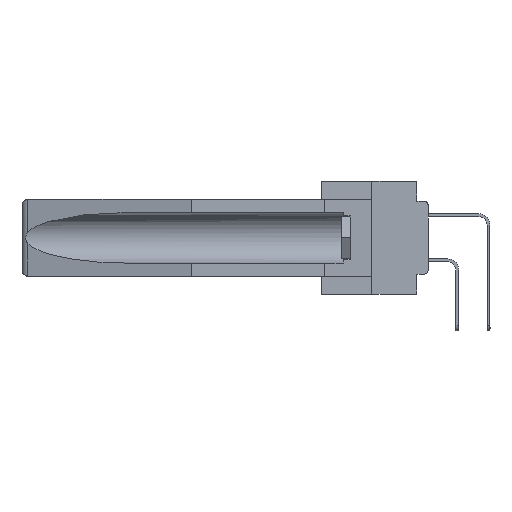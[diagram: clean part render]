
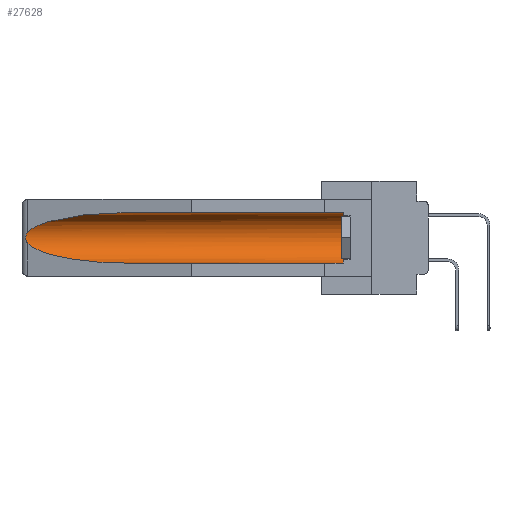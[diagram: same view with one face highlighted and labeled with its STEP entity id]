
A CAD part, left-side view. The second image highlights one B-rep face of the part: STEP entity #27628.
In plain terms, the highlighted cylindrical face has radius 2.857 mm (diameter 5.715 mm), a partial arc.
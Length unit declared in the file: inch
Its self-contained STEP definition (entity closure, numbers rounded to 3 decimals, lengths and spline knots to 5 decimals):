
#10 = ORIENTED_EDGE ( 'NONE', *, *, #17261, .T. ) ;
#563 = CARTESIAN_POINT ( 'NONE',  ( 0.155, -0.30754, -0.059 ) ) ;
#774 = EDGE_CURVE ( 'NONE', #17268, #7400, #1873, .T. ) ;
#1024 = DIRECTION ( 'NONE',  ( 0., 0., 1. ) ) ;
#1674 = CARTESIAN_POINT ( 'NONE',  ( 0.2673, 1.5327, -0.16383 ) ) ;
#1708 = AXIS2_PLACEMENT_3D ( 'NONE', #20218, #1818, #14169 ) ;
#1818 = DIRECTION ( 'NONE',  ( 0., 1., 0. ) ) ;
#1873 =( BOUNDED_CURVE ( )  B_SPLINE_CURVE ( 3, ( #21842, #6467, #18656, #9145 ),
 .UNSPECIFIED., .F., .F. ) 
 B_SPLINE_CURVE_WITH_KNOTS ( ( 4, 4 ),
 ( 4.71239, 6.08839 ),
 .UNSPECIFIED. ) 
 CURVE ( )  GEOMETRIC_REPRESENTATION_ITEM ( )  RATIONAL_B_SPLINE_CURVE ( ( 1., 0.848, 0.848, 1. ) ) 
 REPRESENTATION_ITEM ( '' )  );
#3133 = B_SPLINE_CURVE_WITH_KNOTS ( 'NONE', 3,
 ( #7586, #35607, #32234, #1674, #17251, #38547, #13736, #23155, #4782, #26237 ),
 .UNSPECIFIED., .F., .F.,
 ( 4, 2, 2, 2, 4 ),
 ( 0., 0.00029, 0.00058, 0.00087, 0.00117 ),
 .UNSPECIFIED. ) ;
#3295 = DIRECTION ( 'NONE',  ( 0., 1., 0. ) ) ;
#4119 = CARTESIAN_POINT ( 'NONE',  ( 0.155, 1.07973, -0.059 ) ) ;
#4595 = CARTESIAN_POINT ( 'NONE',  ( 0.155, 1.07973, -0.284 ) ) ;
#4782 = CARTESIAN_POINT ( 'NONE',  ( 0.26597, 1.5296, -0.19026 ) ) ;
#6467 = CARTESIAN_POINT ( 'NONE',  ( 0.21114, 1.30732, -0.059 ) ) ;
#6481 = EDGE_CURVE ( 'NONE', #9315, #17268, #15022, .T. ) ;
#6976 = EDGE_CURVE ( 'NONE', #22000, #14527, #27498, .T. ) ;
#7400 = VERTEX_POINT ( 'NONE', #12946 ) ;
#7586 = CARTESIAN_POINT ( 'NONE',  ( 0.26537, 1.52718, -0.14972 ) ) ;
#8863 = CARTESIAN_POINT ( 'NONE',  ( 0.26537, 1.52718, -0.19328 ) ) ;
#9120 = CARTESIAN_POINT ( 'NONE',  ( 0.155, 1.07973, -0.284 ) ) ;
#9145 = CARTESIAN_POINT ( 'NONE',  ( 0.26537, 1.52718, -0.14972 ) ) ;
#9315 = VERTEX_POINT ( 'NONE', #24206 ) ;
#12233 = ORIENTED_EDGE ( 'NONE', *, *, #31463, .T. ) ;
#12946 = CARTESIAN_POINT ( 'NONE',  ( 0.26537, 1.52718, -0.14972 ) ) ;
#13736 = CARTESIAN_POINT ( 'NONE',  ( 0.2673, 1.53269, -0.17917 ) ) ;
#14034 = VECTOR ( 'NONE', #3295, 39.37008 ) ;
#14169 = DIRECTION ( 'NONE',  ( 0., 0., 1. ) ) ;
#14527 = VERTEX_POINT ( 'NONE', #4595 ) ;
#14904 = VERTEX_POINT ( 'NONE', #16994 ) ;
#15022 = LINE ( 'NONE', #563, #14034 ) ;
#16994 = CARTESIAN_POINT ( 'NONE',  ( 0.26537, 1.52718, -0.19328 ) ) ;
#17251 = CARTESIAN_POINT ( 'NONE',  ( 0.2675, 1.53308, -0.16763 ) ) ;
#17261 = EDGE_CURVE ( 'NONE', #22000, #9315, #21991, .T. ) ;
#17268 = VERTEX_POINT ( 'NONE', #4119 ) ;
#18656 = CARTESIAN_POINT ( 'NONE',  ( 0.25451, 1.48313, -0.09465 ) ) ;
#18945 = AXIS2_PLACEMENT_3D ( 'NONE', #37627, #19433, #1024 ) ;
#19433 = DIRECTION ( 'NONE',  ( 0., -1., 0. ) ) ;
#20218 = CARTESIAN_POINT ( 'NONE',  ( 0.155, -0.30754, -0.1715 ) ) ;
#20818 = CYLINDRICAL_SURFACE ( 'NONE', #1708, 0.1125 ) ;
#21201 = CARTESIAN_POINT ( 'NONE',  ( 0.21114, 1.30732, -0.284 ) ) ;
#21842 = CARTESIAN_POINT ( 'NONE',  ( 0.155, 1.07973, -0.059 ) ) ;
#21991 = CIRCLE ( 'NONE', #18945, 0.1125 ) ;
#22000 = VERTEX_POINT ( 'NONE', #36256 ) ;
#23155 = CARTESIAN_POINT ( 'NONE',  ( 0.26655, 1.53094, -0.18657 ) ) ;
#24119 = DIRECTION ( 'NONE',  ( 0., 1., 0. ) ) ;
#24130 = CARTESIAN_POINT ( 'NONE',  ( 0.25451, 1.48313, -0.24835 ) ) ;
#24206 = CARTESIAN_POINT ( 'NONE',  ( 0.155, 0.126, -0.059 ) ) ;
#25027 = EDGE_LOOP ( 'NONE', ( #36510, #27387, #12233, #37003, #10, #26914 ) ) ;
#25760 = EDGE_CURVE ( 'NONE', #7400, #14904, #3133, .T. ) ;
#26237 = CARTESIAN_POINT ( 'NONE',  ( 0.26537, 1.52718, -0.19328 ) ) ;
#26914 = ORIENTED_EDGE ( 'NONE', *, *, #6481, .T. ) ;
#27387 = ORIENTED_EDGE ( 'NONE', *, *, #25760, .T. ) ;
#27498 = LINE ( 'NONE', #30140, #28881 ) ;
#27628 = ADVANCED_FACE ( 'NONE', ( #32270 ), #20818, .F. ) ;
#28881 = VECTOR ( 'NONE', #24119, 39.37008 ) ;
#30140 = CARTESIAN_POINT ( 'NONE',  ( 0.155, -0.30754, -0.284 ) ) ;
#31463 = EDGE_CURVE ( 'NONE', #14904, #14527, #34052, .T. ) ;
#32234 = CARTESIAN_POINT ( 'NONE',  ( 0.26654, 1.53092, -0.15636 ) ) ;
#32270 = FACE_OUTER_BOUND ( 'NONE', #25027, .T. ) ;
#34052 =( BOUNDED_CURVE ( )  B_SPLINE_CURVE ( 3, ( #8863, #24130, #21201, #9120 ),
 .UNSPECIFIED., .F., .T. ) 
 B_SPLINE_CURVE_WITH_KNOTS ( ( 4, 4 ),
 ( 0.1948, 1.5708 ),
 .UNSPECIFIED. ) 
 CURVE ( )  GEOMETRIC_REPRESENTATION_ITEM ( )  RATIONAL_B_SPLINE_CURVE ( ( 1., 0.848, 0.848, 1. ) ) 
 REPRESENTATION_ITEM ( '' )  );
#35607 = CARTESIAN_POINT ( 'NONE',  ( 0.26597, 1.52961, -0.15275 ) ) ;
#36256 = CARTESIAN_POINT ( 'NONE',  ( 0.155, 0.126, -0.284 ) ) ;
#36510 = ORIENTED_EDGE ( 'NONE', *, *, #774, .T. ) ;
#37003 = ORIENTED_EDGE ( 'NONE', *, *, #6976, .F. ) ;
#37627 = CARTESIAN_POINT ( 'NONE',  ( 0.155, 0.126, -0.1715 ) ) ;
#38547 = CARTESIAN_POINT ( 'NONE',  ( 0.2675, 1.53308, -0.17534 ) ) ;
